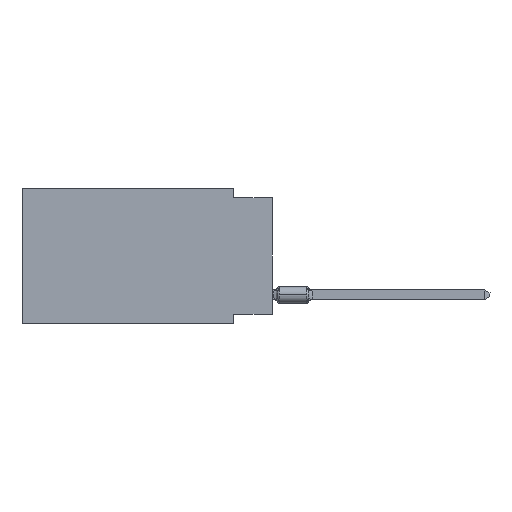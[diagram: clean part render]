
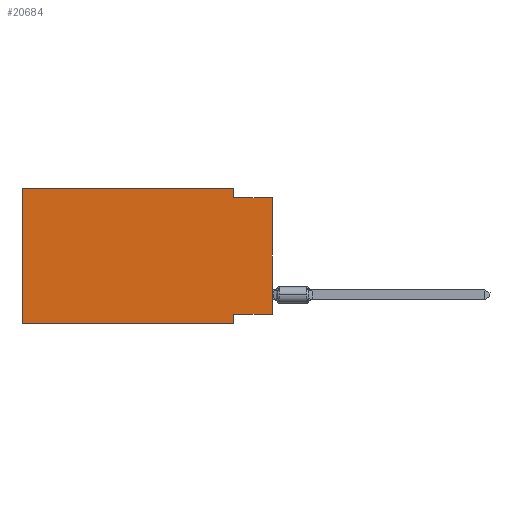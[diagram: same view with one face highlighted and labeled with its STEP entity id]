
A CAD part, left-side view. The second image highlights one B-rep face of the part: STEP entity #20684.
In plain terms, the highlighted planar face has unit normal (-1, 0, 0).
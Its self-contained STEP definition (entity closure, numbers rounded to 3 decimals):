
#560 = EDGE_CURVE ( 'NONE', #3824, #17180, #1345, .T. ) ;
#639 = CARTESIAN_POINT ( 'NONE',  ( 0., 0., -0.635 ) ) ;
#910 = PLANE ( 'NONE',  #6679 ) ;
#1013 = DIRECTION ( 'NONE',  ( 1., 0., 0. ) ) ;
#1345 = LINE ( 'NONE', #23628, #15400 ) ;
#1378 = EDGE_LOOP ( 'NONE', ( #3346, #23078, #21546, #21849, #16384, #20566, #22637, #14796 ) ) ;
#2074 = CARTESIAN_POINT ( 'NONE',  ( 0., 2.54, -8.89 ) ) ;
#3169 = CARTESIAN_POINT ( 'NONE',  ( 0., 2.54, 0. ) ) ;
#3346 = ORIENTED_EDGE ( 'NONE', *, *, #22127, .T. ) ;
#3615 = CARTESIAN_POINT ( 'NONE',  ( 0., 16.383, -8.89 ) ) ;
#3652 = CARTESIAN_POINT ( 'NONE',  ( 0., 2.54, -8.255 ) ) ;
#3824 = VERTEX_POINT ( 'NONE', #19488 ) ;
#3958 = VECTOR ( 'NONE', #13851, 1000. ) ;
#4536 = FACE_OUTER_BOUND ( 'NONE', #1378, .T. ) ;
#5464 = VECTOR ( 'NONE', #21507, 1000. ) ;
#5688 = LINE ( 'NONE', #9663, #23635 ) ;
#5693 = DIRECTION ( 'NONE',  ( 0., 1., 0. ) ) ;
#6679 = AXIS2_PLACEMENT_3D ( 'NONE', #15660, #1013, #8409 ) ;
#7461 = VERTEX_POINT ( 'NONE', #21422 ) ;
#7612 = DIRECTION ( 'NONE',  ( 0., 0., 1. ) ) ;
#7694 = DIRECTION ( 'NONE',  ( 0., 0., 1. ) ) ;
#8299 = LINE ( 'NONE', #19175, #3958 ) ;
#8409 = DIRECTION ( 'NONE',  ( 0., 0., -1. ) ) ;
#9236 = CARTESIAN_POINT ( 'NONE',  ( 0., 2.54, -8.89 ) ) ;
#9663 = CARTESIAN_POINT ( 'NONE',  ( 0., 16.383, 0. ) ) ;
#9982 = VECTOR ( 'NONE', #16474, 1000. ) ;
#11128 = CARTESIAN_POINT ( 'NONE',  ( 0., 2.54, 0. ) ) ;
#11252 = VERTEX_POINT ( 'NONE', #3169 ) ;
#12881 = VERTEX_POINT ( 'NONE', #23721 ) ;
#13851 = DIRECTION ( 'NONE',  ( 0., -1., 0. ) ) ;
#13995 = VECTOR ( 'NONE', #19961, 1000. ) ;
#13997 = EDGE_CURVE ( 'NONE', #20405, #7461, #5688, .T. ) ;
#14025 = VECTOR ( 'NONE', #15398, 1000. ) ;
#14056 = VECTOR ( 'NONE', #7694, 1000. ) ;
#14796 = ORIENTED_EDGE ( 'NONE', *, *, #560, .F. ) ;
#14980 = EDGE_CURVE ( 'NONE', #7461, #11252, #20202, .T. ) ;
#15398 = DIRECTION ( 'NONE',  ( 0., -1., 0. ) ) ;
#15400 = VECTOR ( 'NONE', #5693, 1000. ) ;
#15660 = CARTESIAN_POINT ( 'NONE',  ( 0., 16.383, 0. ) ) ;
#16333 = LINE ( 'NONE', #11128, #13995 ) ;
#16384 = ORIENTED_EDGE ( 'NONE', *, *, #13997, .F. ) ;
#16474 = DIRECTION ( 'NONE',  ( 0., 0., -1. ) ) ;
#17180 = VERTEX_POINT ( 'NONE', #3652 ) ;
#17210 = VERTEX_POINT ( 'NONE', #2074 ) ;
#17213 = LINE ( 'NONE', #639, #14025 ) ;
#18318 = EDGE_CURVE ( 'NONE', #20405, #17210, #8299, .T. ) ;
#18356 = CARTESIAN_POINT ( 'NONE',  ( 0., 0., 0. ) ) ;
#18809 = LINE ( 'NONE', #18356, #14056 ) ;
#18822 = EDGE_CURVE ( 'NONE', #11252, #19571, #16333, .T. ) ;
#19175 = CARTESIAN_POINT ( 'NONE',  ( 0., 16.383, -8.89 ) ) ;
#19488 = CARTESIAN_POINT ( 'NONE',  ( 0., 0., -8.255 ) ) ;
#19571 = VERTEX_POINT ( 'NONE', #22085 ) ;
#19961 = DIRECTION ( 'NONE',  ( 0., 0., -1. ) ) ;
#20202 = LINE ( 'NONE', #21646, #5464 ) ;
#20405 = VERTEX_POINT ( 'NONE', #3615 ) ;
#20566 = ORIENTED_EDGE ( 'NONE', *, *, #18318, .T. ) ;
#20684 = ADVANCED_FACE ( 'NONE', ( #4536 ), #910, .F. ) ;
#21065 = EDGE_CURVE ( 'NONE', #19571, #12881, #17213, .T. ) ;
#21422 = CARTESIAN_POINT ( 'NONE',  ( 0., 16.383, 0. ) ) ;
#21507 = DIRECTION ( 'NONE',  ( 0., -1., 0. ) ) ;
#21546 = ORIENTED_EDGE ( 'NONE', *, *, #18822, .F. ) ;
#21646 = CARTESIAN_POINT ( 'NONE',  ( 0., 16.383, 0. ) ) ;
#21849 = ORIENTED_EDGE ( 'NONE', *, *, #14980, .F. ) ;
#22085 = CARTESIAN_POINT ( 'NONE',  ( 0., 2.54, -0.635 ) ) ;
#22127 = EDGE_CURVE ( 'NONE', #3824, #12881, #18809, .T. ) ;
#22417 = LINE ( 'NONE', #9236, #9982 ) ;
#22513 = EDGE_CURVE ( 'NONE', #17180, #17210, #22417, .T. ) ;
#22637 = ORIENTED_EDGE ( 'NONE', *, *, #22513, .F. ) ;
#23078 = ORIENTED_EDGE ( 'NONE', *, *, #21065, .F. ) ;
#23628 = CARTESIAN_POINT ( 'NONE',  ( 0., 0., -8.255 ) ) ;
#23635 = VECTOR ( 'NONE', #7612, 1000. ) ;
#23721 = CARTESIAN_POINT ( 'NONE',  ( 0., 0., -0.635 ) ) ;
